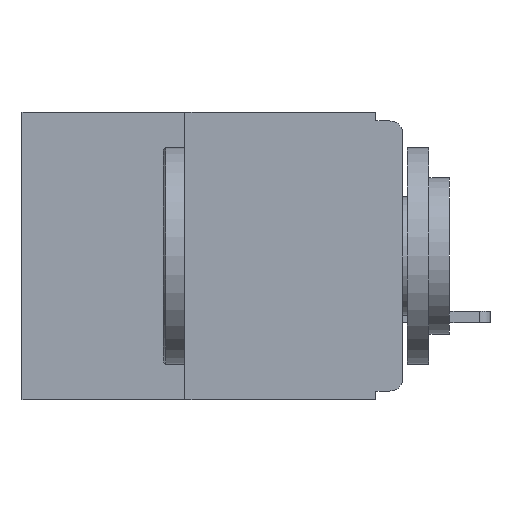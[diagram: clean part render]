
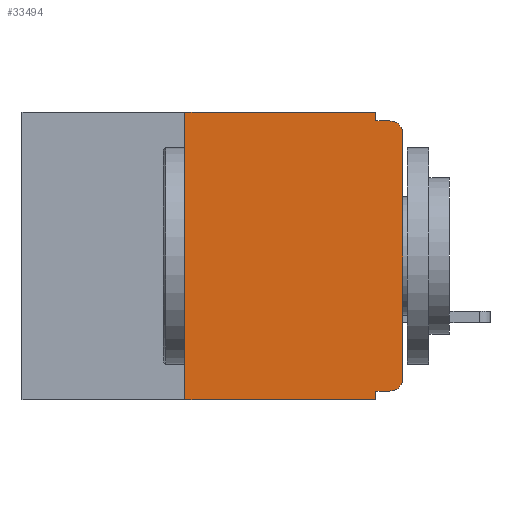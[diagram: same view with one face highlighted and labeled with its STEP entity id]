
A CAD part, left-side view. The second image highlights one B-rep face of the part: STEP entity #33494.
In plain terms, the highlighted planar face has unit normal (-1, 0, 0).
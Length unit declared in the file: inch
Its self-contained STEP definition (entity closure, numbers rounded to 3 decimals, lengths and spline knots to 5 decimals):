
#835 = PLANE ( 'NONE',  #19096 ) ;
#955 = DIRECTION ( 'NONE',  ( 1., 0., 0. ) ) ;
#1422 = CARTESIAN_POINT ( 'NONE',  ( 0., 0.031, -0.33 ) ) ;
#1507 = LINE ( 'NONE', #33840, #8962 ) ;
#1754 = ORIENTED_EDGE ( 'NONE', *, *, #25931, .T. ) ;
#1870 = DIRECTION ( 'NONE',  ( 0., 0., -1. ) ) ;
#1916 = CARTESIAN_POINT ( 'NONE',  ( 0., 0., -0.32 ) ) ;
#2008 = VECTOR ( 'NONE', #30065, 39.37008 ) ;
#2541 = EDGE_CURVE ( 'NONE', #25729, #27453, #29879, .T. ) ;
#3177 = CARTESIAN_POINT ( 'NONE',  ( 0., 0.015, -0.025 ) ) ;
#3235 = EDGE_CURVE ( 'NONE', #20210, #19367, #16653, .T. ) ;
#3508 = DIRECTION ( 'NONE',  ( 0., 0., 1. ) ) ;
#3595 = CARTESIAN_POINT ( 'NONE',  ( 0., 0.25, -0.33 ) ) ;
#3957 = EDGE_CURVE ( 'NONE', #29909, #11494, #1507, .T. ) ;
#4843 = CARTESIAN_POINT ( 'NONE',  ( 0., 0.25, -0.33 ) ) ;
#5771 = EDGE_CURVE ( 'NONE', #20210, #25729, #27294, .T. ) ;
#6004 = DIRECTION ( 'NONE',  ( 0., 0., -1. ) ) ;
#6053 = CARTESIAN_POINT ( 'NONE',  ( 0., 0.015, -0.01 ) ) ;
#7400 = ORIENTED_EDGE ( 'NONE', *, *, #8219, .F. ) ;
#7418 = CARTESIAN_POINT ( 'NONE',  ( 0., 0., -0.305 ) ) ;
#8219 = EDGE_CURVE ( 'NONE', #23958, #19367, #25857, .T. ) ;
#8340 = EDGE_CURVE ( 'NONE', #25025, #23958, #10002, .T. ) ;
#8962 = VECTOR ( 'NONE', #33399, 39.37008 ) ;
#8974 = EDGE_CURVE ( 'NONE', #27453, #13478, #15872, .T. ) ;
#9371 = ORIENTED_EDGE ( 'NONE', *, *, #2541, .F. ) ;
#9747 = CARTESIAN_POINT ( 'NONE',  ( 0., 0.031, 0. ) ) ;
#10002 = LINE ( 'NONE', #1916, #14663 ) ;
#10894 = ORIENTED_EDGE ( 'NONE', *, *, #3957, .T. ) ;
#11439 = ORIENTED_EDGE ( 'NONE', *, *, #8340, .F. ) ;
#11494 = VERTEX_POINT ( 'NONE', #14707 ) ;
#11815 = AXIS2_PLACEMENT_3D ( 'NONE', #29699, #13834, #32316 ) ;
#12440 = VECTOR ( 'NONE', #17523, 39.37008 ) ;
#12481 = DIRECTION ( 'NONE',  ( 0., 0., -1. ) ) ;
#13153 = VECTOR ( 'NONE', #3508, 39.37008 ) ;
#13478 = VERTEX_POINT ( 'NONE', #34866 ) ;
#13834 = DIRECTION ( 'NONE',  ( -1., 0., 0. ) ) ;
#14663 = VECTOR ( 'NONE', #15671, 39.37008 ) ;
#14707 = CARTESIAN_POINT ( 'NONE',  ( 0., 0., -0.025 ) ) ;
#15671 = DIRECTION ( 'NONE',  ( 0., 1., 0. ) ) ;
#15817 = VECTOR ( 'NONE', #29328, 39.37008 ) ;
#15872 = LINE ( 'NONE', #31574, #22074 ) ;
#15874 = ORIENTED_EDGE ( 'NONE', *, *, #25826, .T. ) ;
#15950 = CARTESIAN_POINT ( 'NONE',  ( 0., 0.031, -0.32 ) ) ;
#16331 = CIRCLE ( 'NONE', #11815, 0.015 ) ;
#16653 = LINE ( 'NONE', #30327, #2008 ) ;
#17523 = DIRECTION ( 'NONE',  ( 0., -1., 0. ) ) ;
#18057 = ORIENTED_EDGE ( 'NONE', *, *, #5771, .F. ) ;
#18352 = CARTESIAN_POINT ( 'NONE',  ( 0., 0.015, -0.32 ) ) ;
#19096 = AXIS2_PLACEMENT_3D ( 'NONE', #30627, #955, #20125 ) ;
#19367 = VERTEX_POINT ( 'NONE', #19984 ) ;
#19984 = CARTESIAN_POINT ( 'NONE',  ( 0., 0.031, -0.33 ) ) ;
#20056 = CIRCLE ( 'NONE', #20810, 0.015 ) ;
#20125 = DIRECTION ( 'NONE',  ( 0., 0., -1. ) ) ;
#20210 = VERTEX_POINT ( 'NONE', #4843 ) ;
#20810 = AXIS2_PLACEMENT_3D ( 'NONE', #3177, #22181, #6004 ) ;
#21008 = ORIENTED_EDGE ( 'NONE', *, *, #8974, .F. ) ;
#21484 = EDGE_CURVE ( 'NONE', #13478, #27842, #26608, .T. ) ;
#22074 = VECTOR ( 'NONE', #1870, 39.37008 ) ;
#22181 = DIRECTION ( 'NONE',  ( -1., 0., 0. ) ) ;
#22736 = CARTESIAN_POINT ( 'NONE',  ( 0., 0., -0.01 ) ) ;
#23958 = VERTEX_POINT ( 'NONE', #15950 ) ;
#25021 = FACE_OUTER_BOUND ( 'NONE', #26063, .T. ) ;
#25025 = VERTEX_POINT ( 'NONE', #18352 ) ;
#25729 = VERTEX_POINT ( 'NONE', #29257 ) ;
#25826 = EDGE_CURVE ( 'NONE', #25025, #29909, #16331, .T. ) ;
#25857 = LINE ( 'NONE', #1422, #32827 ) ;
#25931 = EDGE_CURVE ( 'NONE', #11494, #27842, #20056, .T. ) ;
#26063 = EDGE_LOOP ( 'NONE', ( #10894, #1754, #32586, #21008, #9371, #18057, #34158, #7400, #11439, #15874 ) ) ;
#26608 = LINE ( 'NONE', #22736, #12440 ) ;
#27294 = LINE ( 'NONE', #3595, #13153 ) ;
#27453 = VERTEX_POINT ( 'NONE', #9747 ) ;
#27842 = VERTEX_POINT ( 'NONE', #6053 ) ;
#29257 = CARTESIAN_POINT ( 'NONE',  ( 0., 0.25, 0. ) ) ;
#29328 = DIRECTION ( 'NONE',  ( 0., -1., 0. ) ) ;
#29699 = CARTESIAN_POINT ( 'NONE',  ( 0., 0.015, -0.305 ) ) ;
#29879 = LINE ( 'NONE', #31310, #15817 ) ;
#29909 = VERTEX_POINT ( 'NONE', #7418 ) ;
#30065 = DIRECTION ( 'NONE',  ( 0., -1., 0. ) ) ;
#30327 = CARTESIAN_POINT ( 'NONE',  ( 0., 0.437, -0.33 ) ) ;
#30627 = CARTESIAN_POINT ( 'NONE',  ( 0., 0.437, 0. ) ) ;
#31310 = CARTESIAN_POINT ( 'NONE',  ( 0., 0.437, 0. ) ) ;
#31574 = CARTESIAN_POINT ( 'NONE',  ( 0., 0.031, 0. ) ) ;
#32316 = DIRECTION ( 'NONE',  ( 0., 0., -1. ) ) ;
#32586 = ORIENTED_EDGE ( 'NONE', *, *, #21484, .F. ) ;
#32827 = VECTOR ( 'NONE', #12481, 39.37008 ) ;
#33399 = DIRECTION ( 'NONE',  ( 0., 0., 1. ) ) ;
#33494 = ADVANCED_FACE ( 'NONE', ( #25021 ), #835, .F. ) ;
#33840 = CARTESIAN_POINT ( 'NONE',  ( 0., 0., 0. ) ) ;
#34158 = ORIENTED_EDGE ( 'NONE', *, *, #3235, .T. ) ;
#34866 = CARTESIAN_POINT ( 'NONE',  ( 0., 0.031, -0.01 ) ) ;
